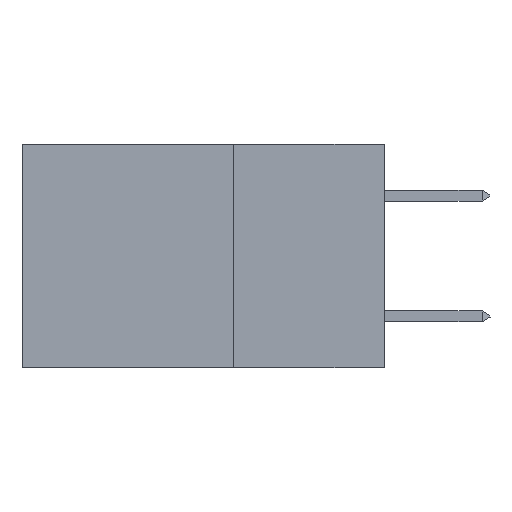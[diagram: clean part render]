
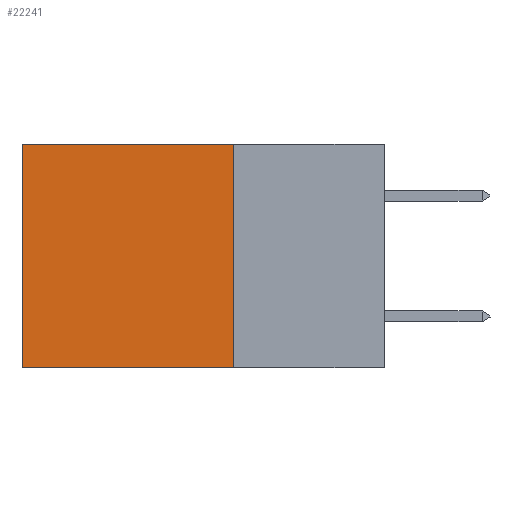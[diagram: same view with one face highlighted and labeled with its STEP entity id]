
A CAD part, left-side view. The second image highlights one B-rep face of the part: STEP entity #22241.
In plain terms, the highlighted planar face has unit normal (-1, 0, 0).
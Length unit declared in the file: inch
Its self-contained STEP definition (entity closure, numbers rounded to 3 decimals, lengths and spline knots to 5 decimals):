
#242 = CARTESIAN_POINT ( 'NONE',  ( 0.2875, 0.25, 0. ) ) ;
#2136 = VERTEX_POINT ( 'NONE', #22151 ) ;
#3185 = CARTESIAN_POINT ( 'NONE',  ( 0.2875, 0.25, 0. ) ) ;
#3620 = ORIENTED_EDGE ( 'NONE', *, *, #29189, .F. ) ;
#4118 = AXIS2_PLACEMENT_3D ( 'NONE', #12997, #17512, #15331 ) ;
#8079 = VECTOR ( 'NONE', #17794, 39.37008 ) ;
#8652 = VERTEX_POINT ( 'NONE', #15517 ) ;
#9105 = VECTOR ( 'NONE', #10714, 39.37008 ) ;
#10714 = DIRECTION ( 'NONE',  ( 0., 1., 0. ) ) ;
#12664 = LINE ( 'NONE', #16992, #30006 ) ;
#12997 = CARTESIAN_POINT ( 'NONE',  ( 0.2875, 0.25, 0. ) ) ;
#13654 = EDGE_LOOP ( 'NONE', ( #15882, #3620, #14441, #26021 ) ) ;
#14358 = VERTEX_POINT ( 'NONE', #242 ) ;
#14441 = ORIENTED_EDGE ( 'NONE', *, *, #15914, .F. ) ;
#15331 = DIRECTION ( 'NONE',  ( 0., 0., -1. ) ) ;
#15517 = CARTESIAN_POINT ( 'NONE',  ( 0.2875, 0.6, -0.37 ) ) ;
#15882 = ORIENTED_EDGE ( 'NONE', *, *, #21991, .T. ) ;
#15914 = EDGE_CURVE ( 'NONE', #14358, #2136, #22002, .T. ) ;
#16077 = CARTESIAN_POINT ( 'NONE',  ( 0.2875, 0.6, 0. ) ) ;
#16992 = CARTESIAN_POINT ( 'NONE',  ( 0.2875, 0.25, -0.37 ) ) ;
#17512 = DIRECTION ( 'NONE',  ( 1., 0., 0. ) ) ;
#17604 = DIRECTION ( 'NONE',  ( 0., 0., -1. ) ) ;
#17794 = DIRECTION ( 'NONE',  ( 0., 0., -1. ) ) ;
#18494 = DIRECTION ( 'NONE',  ( 0., 1., 0. ) ) ;
#18971 = VECTOR ( 'NONE', #17604, 39.37008 ) ;
#19876 = PLANE ( 'NONE',  #4118 ) ;
#19970 = CARTESIAN_POINT ( 'NONE',  ( 0.2875, 0.25, 0. ) ) ;
#21553 = LINE ( 'NONE', #3185, #9105 ) ;
#21991 = EDGE_CURVE ( 'NONE', #30135, #8652, #24252, .T. ) ;
#22002 = LINE ( 'NONE', #19970, #18971 ) ;
#22151 = CARTESIAN_POINT ( 'NONE',  ( 0.2875, 0.25, -0.37 ) ) ;
#22241 = ADVANCED_FACE ( 'NONE', ( #30301 ), #19876, .F. ) ;
#24252 = LINE ( 'NONE', #28290, #8079 ) ;
#26021 = ORIENTED_EDGE ( 'NONE', *, *, #26288, .T. ) ;
#26288 = EDGE_CURVE ( 'NONE', #14358, #30135, #21553, .T. ) ;
#28290 = CARTESIAN_POINT ( 'NONE',  ( 0.2875, 0.6, 0. ) ) ;
#29189 = EDGE_CURVE ( 'NONE', #2136, #8652, #12664, .T. ) ;
#30006 = VECTOR ( 'NONE', #18494, 39.37008 ) ;
#30135 = VERTEX_POINT ( 'NONE', #16077 ) ;
#30301 = FACE_OUTER_BOUND ( 'NONE', #13654, .T. ) ;
